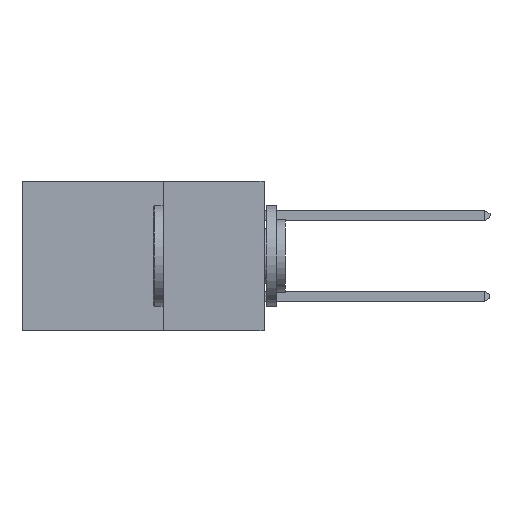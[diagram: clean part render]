
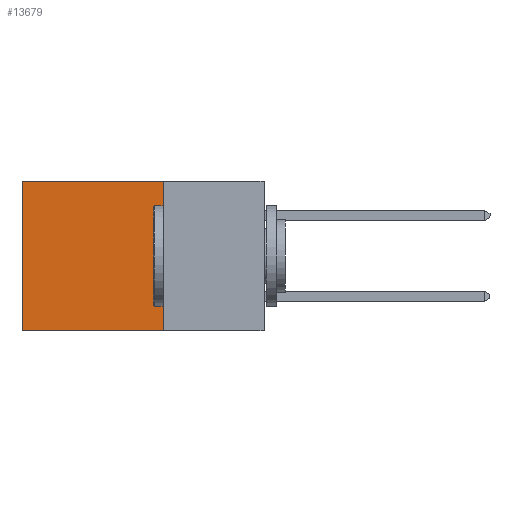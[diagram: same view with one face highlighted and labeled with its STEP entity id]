
A CAD part, left-side view. The second image highlights one B-rep face of the part: STEP entity #13679.
In plain terms, the highlighted planar face has unit normal (-1, 0, 0).
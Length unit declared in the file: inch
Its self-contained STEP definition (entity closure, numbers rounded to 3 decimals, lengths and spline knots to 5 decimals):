
#137 = ORIENTED_EDGE ( 'NONE', *, *, #3806, .T. ) ;
#249 = VECTOR ( 'NONE', #10574, 39.37008 ) ;
#688 = DIRECTION ( 'NONE',  ( 0., 0., -1. ) ) ;
#1892 = CARTESIAN_POINT ( 'NONE',  ( 0.298, 0.25, 0. ) ) ;
#1975 = EDGE_CURVE ( 'NONE', #2035, #3621, #8188, .T. ) ;
#2035 = VERTEX_POINT ( 'NONE', #1892 ) ;
#2480 = CARTESIAN_POINT ( 'NONE',  ( 0.298, 0.25, 0. ) ) ;
#2871 = ORIENTED_EDGE ( 'NONE', *, *, #3318, .T. ) ;
#3303 = VERTEX_POINT ( 'NONE', #13954 ) ;
#3318 = EDGE_CURVE ( 'NONE', #2035, #3303, #6950, .T. ) ;
#3621 = VERTEX_POINT ( 'NONE', #15477 ) ;
#3806 = EDGE_CURVE ( 'NONE', #3303, #9213, #3884, .T. ) ;
#3884 = LINE ( 'NONE', #11834, #249 ) ;
#4958 = VECTOR ( 'NONE', #7654, 39.37008 ) ;
#6817 = PLANE ( 'NONE',  #11761 ) ;
#6853 = CARTESIAN_POINT ( 'NONE',  ( 0.298, 0.6, -0.37 ) ) ;
#6950 = LINE ( 'NONE', #14261, #13501 ) ;
#7654 = DIRECTION ( 'NONE',  ( 0., 1., 0. ) ) ;
#8076 = DIRECTION ( 'NONE',  ( 1., 0., 0. ) ) ;
#8188 = LINE ( 'NONE', #2480, #15044 ) ;
#8256 = LINE ( 'NONE', #10124, #4958 ) ;
#9213 = VERTEX_POINT ( 'NONE', #6853 ) ;
#9340 = EDGE_LOOP ( 'NONE', ( #137, #13590, #13116, #2871 ) ) ;
#10124 = CARTESIAN_POINT ( 'NONE',  ( 0.298, 0.25, -0.37 ) ) ;
#10147 = DIRECTION ( 'NONE',  ( 0., 0., -1. ) ) ;
#10574 = DIRECTION ( 'NONE',  ( 0., 0., -1. ) ) ;
#11761 = AXIS2_PLACEMENT_3D ( 'NONE', #14167, #8076, #688 ) ;
#11834 = CARTESIAN_POINT ( 'NONE',  ( 0.298, 0.6, 0. ) ) ;
#13116 = ORIENTED_EDGE ( 'NONE', *, *, #1975, .F. ) ;
#13490 = EDGE_CURVE ( 'NONE', #3621, #9213, #8256, .T. ) ;
#13501 = VECTOR ( 'NONE', #15166, 39.37008 ) ;
#13590 = ORIENTED_EDGE ( 'NONE', *, *, #13490, .F. ) ;
#13679 = ADVANCED_FACE ( 'NONE', ( #14911 ), #6817, .F. ) ;
#13954 = CARTESIAN_POINT ( 'NONE',  ( 0.298, 0.6, 0. ) ) ;
#14167 = CARTESIAN_POINT ( 'NONE',  ( 0.298, 0.25, 0. ) ) ;
#14261 = CARTESIAN_POINT ( 'NONE',  ( 0.298, 0.25, 0. ) ) ;
#14911 = FACE_OUTER_BOUND ( 'NONE', #9340, .T. ) ;
#15044 = VECTOR ( 'NONE', #10147, 39.37008 ) ;
#15166 = DIRECTION ( 'NONE',  ( 0., 1., 0. ) ) ;
#15477 = CARTESIAN_POINT ( 'NONE',  ( 0.298, 0.25, -0.37 ) ) ;
